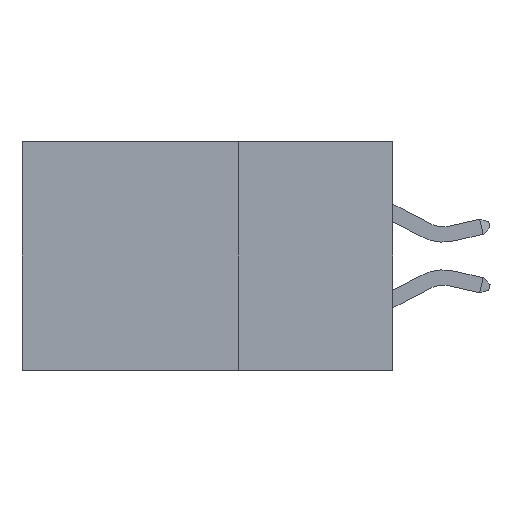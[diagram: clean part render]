
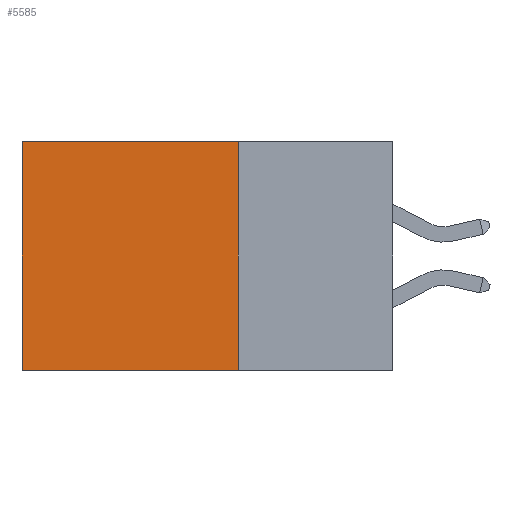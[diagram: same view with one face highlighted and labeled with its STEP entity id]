
A CAD part, left-side view. The second image highlights one B-rep face of the part: STEP entity #5585.
In plain terms, the highlighted planar face has unit normal (-1, 0, 0).
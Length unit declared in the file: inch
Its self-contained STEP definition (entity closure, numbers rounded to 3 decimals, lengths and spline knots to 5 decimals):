
#336 = EDGE_LOOP ( 'NONE', ( #9072, #13106, #13930, #17503 ) ) ;
#881 = VECTOR ( 'NONE', #9906, 39.37008 ) ;
#1222 = CARTESIAN_POINT ( 'NONE',  ( 0.2875, 0.25, -0.37 ) ) ;
#2001 = FACE_OUTER_BOUND ( 'NONE', #336, .T. ) ;
#2511 = CARTESIAN_POINT ( 'NONE',  ( 0.2875, 0.6, -0.37 ) ) ;
#3427 = VERTEX_POINT ( 'NONE', #17557 ) ;
#3707 = DIRECTION ( 'NONE',  ( 0., 0., -1. ) ) ;
#3756 = VERTEX_POINT ( 'NONE', #13155 ) ;
#4748 = CARTESIAN_POINT ( 'NONE',  ( 0.2875, 0.25, 0. ) ) ;
#4809 = AXIS2_PLACEMENT_3D ( 'NONE', #13270, #12023, #3707 ) ;
#4934 = VECTOR ( 'NONE', #8897, 39.37008 ) ;
#5585 = ADVANCED_FACE ( 'NONE', ( #2001 ), #10684, .F. ) ;
#7195 = EDGE_CURVE ( 'NONE', #3756, #10111, #17079, .T. ) ;
#7500 = LINE ( 'NONE', #14719, #17914 ) ;
#8620 = VERTEX_POINT ( 'NONE', #14156 ) ;
#8897 = DIRECTION ( 'NONE',  ( 0., 0., -1. ) ) ;
#9072 = ORIENTED_EDGE ( 'NONE', *, *, #7195, .T. ) ;
#9819 = DIRECTION ( 'NONE',  ( 0., 0., -1. ) ) ;
#9906 = DIRECTION ( 'NONE',  ( 0., 1., 0. ) ) ;
#10111 = VERTEX_POINT ( 'NONE', #2511 ) ;
#10252 = EDGE_CURVE ( 'NONE', #8620, #10111, #12281, .T. ) ;
#10684 = PLANE ( 'NONE',  #4809 ) ;
#11331 = EDGE_CURVE ( 'NONE', #3427, #8620, #14950, .T. ) ;
#11565 = EDGE_CURVE ( 'NONE', #3427, #3756, #7500, .T. ) ;
#12023 = DIRECTION ( 'NONE',  ( 1., 0., 0. ) ) ;
#12281 = LINE ( 'NONE', #1222, #881 ) ;
#13106 = ORIENTED_EDGE ( 'NONE', *, *, #10252, .F. ) ;
#13155 = CARTESIAN_POINT ( 'NONE',  ( 0.2875, 0.6, 0. ) ) ;
#13270 = CARTESIAN_POINT ( 'NONE',  ( 0.2875, 0.25, 0. ) ) ;
#13839 = CARTESIAN_POINT ( 'NONE',  ( 0.2875, 0.6, 0. ) ) ;
#13930 = ORIENTED_EDGE ( 'NONE', *, *, #11331, .F. ) ;
#14156 = CARTESIAN_POINT ( 'NONE',  ( 0.2875, 0.25, -0.37 ) ) ;
#14676 = VECTOR ( 'NONE', #9819, 39.37008 ) ;
#14719 = CARTESIAN_POINT ( 'NONE',  ( 0.2875, 0.25, 0. ) ) ;
#14950 = LINE ( 'NONE', #4748, #4934 ) ;
#17079 = LINE ( 'NONE', #13839, #14676 ) ;
#17415 = DIRECTION ( 'NONE',  ( 0., 1., 0. ) ) ;
#17503 = ORIENTED_EDGE ( 'NONE', *, *, #11565, .T. ) ;
#17557 = CARTESIAN_POINT ( 'NONE',  ( 0.2875, 0.25, 0. ) ) ;
#17914 = VECTOR ( 'NONE', #17415, 39.37008 ) ;
